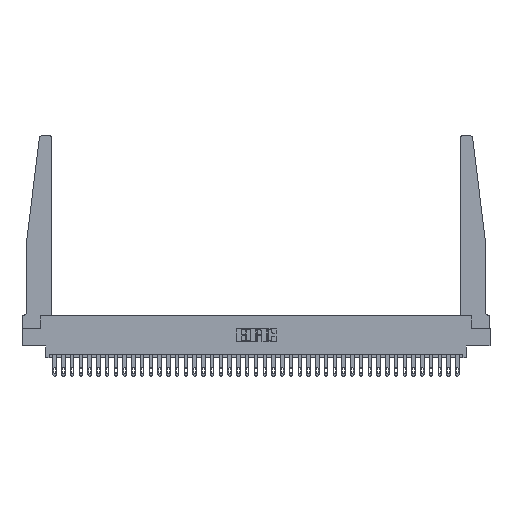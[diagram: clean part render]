
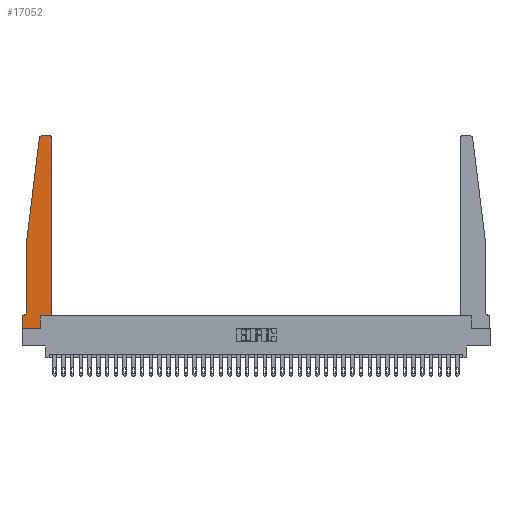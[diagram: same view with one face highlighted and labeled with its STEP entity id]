
A CAD part, top view. The second image highlights one B-rep face of the part: STEP entity #17052.
In plain terms, the highlighted planar face has unit normal (0, 0, 1).
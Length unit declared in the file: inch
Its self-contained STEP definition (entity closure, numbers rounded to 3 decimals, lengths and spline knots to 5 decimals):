
#277 = CARTESIAN_POINT ( 'NONE',  ( 0., 0.1875, 0.37 ) ) ;
#583 = CARTESIAN_POINT ( 'NONE',  ( 0., 0., 0.37 ) ) ;
#2379 = DIRECTION ( 'NONE',  ( 1., 0., 0. ) ) ;
#2888 = AXIS2_PLACEMENT_3D ( 'NONE', #5054, #20928, #2379 ) ;
#2895 = LINE ( 'NONE', #10766, #8839 ) ;
#2962 = EDGE_CURVE ( 'NONE', #16837, #6797, #2895, .T. ) ;
#3125 = VERTEX_POINT ( 'NONE', #22333 ) ;
#3218 = VERTEX_POINT ( 'NONE', #14650 ) ;
#3369 = DIRECTION ( 'NONE',  ( -1., 0., 0. ) ) ;
#3624 = EDGE_CURVE ( 'NONE', #3125, #34445, #22843, .T. ) ;
#4227 = LINE ( 'NONE', #7274, #10777 ) ;
#4383 = EDGE_CURVE ( 'NONE', #6797, #17259, #32723, .T. ) ;
#4899 = DIRECTION ( 'NONE',  ( 1., 0., 0. ) ) ;
#4927 = EDGE_CURVE ( 'NONE', #32567, #3218, #4227, .T. ) ;
#5054 = CARTESIAN_POINT ( 'NONE',  ( 0., 0.1875, 0.37 ) ) ;
#5168 = CARTESIAN_POINT ( 'NONE',  ( 0.015, 0.1875, 0.37 ) ) ;
#5901 = AXIS2_PLACEMENT_3D ( 'NONE', #31865, #12219, #31333 ) ;
#6479 = VECTOR ( 'NONE', #4899, 39.37008 ) ;
#6797 = VERTEX_POINT ( 'NONE', #9288 ) ;
#7006 = EDGE_CURVE ( 'NONE', #24190, #20669, #18581, .T. ) ;
#7035 = VECTOR ( 'NONE', #25612, 39.37008 ) ;
#7226 = CARTESIAN_POINT ( 'NONE',  ( 0.065, 1.25, 0.37 ) ) ;
#7274 = CARTESIAN_POINT ( 'NONE',  ( 0.25, 2.75, 0.37 ) ) ;
#7833 = ORIENTED_EDGE ( 'NONE', *, *, #18658, .T. ) ;
#8265 = AXIS2_PLACEMENT_3D ( 'NONE', #8854, #23119, #19753 ) ;
#8781 = EDGE_LOOP ( 'NONE', ( #22103, #17654, #23319, #31981, #24513, #7833, #25959, #12673, #13867, #21754, #24614, #31570 ) ) ;
#8839 = VECTOR ( 'NONE', #32549, 39.37008 ) ;
#8854 = CARTESIAN_POINT ( 'NONE',  ( 0.27653, 2.72, 0.37 ) ) ;
#9288 = CARTESIAN_POINT ( 'NONE',  ( 0.2605, 0., 0.37 ) ) ;
#10540 = CARTESIAN_POINT ( 'NONE',  ( 0.015, 0.2375, 0.37 ) ) ;
#10766 = CARTESIAN_POINT ( 'NONE',  ( 0., 0., 0.37 ) ) ;
#10777 = VECTOR ( 'NONE', #15133, 39.37008 ) ;
#12219 = DIRECTION ( 'NONE',  ( 0., 0., 1. ) ) ;
#12673 = ORIENTED_EDGE ( 'NONE', *, *, #2962, .T. ) ;
#12890 = EDGE_CURVE ( 'NONE', #15162, #16837, #29747, .T. ) ;
#13042 = CARTESIAN_POINT ( 'NONE',  ( 0.395, 2.75, 0.37 ) ) ;
#13258 = CARTESIAN_POINT ( 'NONE',  ( 0.2605, 0.18, 0.37 ) ) ;
#13793 = VECTOR ( 'NONE', #25829, 39.37008 ) ;
#13867 = ORIENTED_EDGE ( 'NONE', *, *, #4383, .T. ) ;
#14650 = CARTESIAN_POINT ( 'NONE',  ( 0.27653, 2.75, 0.37 ) ) ;
#14926 = CARTESIAN_POINT ( 'NONE',  ( 0.065, 1.25, 0.37 ) ) ;
#14945 = LINE ( 'NONE', #15122, #13793 ) ;
#15040 = VECTOR ( 'NONE', #29284, 39.37008 ) ;
#15122 = CARTESIAN_POINT ( 'NONE',  ( 0.065, 0.1875, 0.37 ) ) ;
#15133 = DIRECTION ( 'NONE',  ( -1., 0., 0. ) ) ;
#15162 = VERTEX_POINT ( 'NONE', #277 ) ;
#16837 = VERTEX_POINT ( 'NONE', #583 ) ;
#17052 = ADVANCED_FACE ( 'NONE', ( #29517 ), #20581, .T. ) ;
#17090 = VECTOR ( 'NONE', #24504, 39.37008 ) ;
#17259 = VERTEX_POINT ( 'NONE', #18975 ) ;
#17425 = LINE ( 'NONE', #14926, #28776 ) ;
#17654 = ORIENTED_EDGE ( 'NONE', *, *, #22647, .T. ) ;
#17788 = CARTESIAN_POINT ( 'NONE',  ( 0.24675, 2.72367, 0.37 ) ) ;
#18114 = LINE ( 'NONE', #7226, #7035 ) ;
#18581 = LINE ( 'NONE', #23205, #15040 ) ;
#18658 = EDGE_CURVE ( 'NONE', #34445, #15162, #14945, .T. ) ;
#18975 = CARTESIAN_POINT ( 'NONE',  ( 0.2605, 0.18, 0.37 ) ) ;
#19169 = EDGE_CURVE ( 'NONE', #17259, #24190, #32034, .T. ) ;
#19753 = DIRECTION ( 'NONE',  ( 1., 0., 0. ) ) ;
#19974 = DIRECTION ( 'NONE',  ( 0., 0., -1. ) ) ;
#20311 = EDGE_CURVE ( 'NONE', #34511, #3125, #18114, .T. ) ;
#20425 = EDGE_CURVE ( 'NONE', #20669, #32567, #25247, .T. ) ;
#20581 = PLANE ( 'NONE',  #2888 ) ;
#20669 = VERTEX_POINT ( 'NONE', #24692 ) ;
#20928 = DIRECTION ( 'NONE',  ( 0., 0., 1. ) ) ;
#21522 = CARTESIAN_POINT ( 'NONE',  ( 0., 0., 0.37 ) ) ;
#21666 = CARTESIAN_POINT ( 'NONE',  ( 0.425, 0.18, 0.37 ) ) ;
#21754 = ORIENTED_EDGE ( 'NONE', *, *, #19169, .T. ) ;
#22103 = ORIENTED_EDGE ( 'NONE', *, *, #4927, .T. ) ;
#22333 = CARTESIAN_POINT ( 'NONE',  ( 0.065, 0.2375, 0.37 ) ) ;
#22647 = EDGE_CURVE ( 'NONE', #3218, #26570, #23637, .T. ) ;
#22843 = CIRCLE ( 'NONE', #27419, 0.05 ) ;
#23119 = DIRECTION ( 'NONE',  ( 0., 0., 1. ) ) ;
#23205 = CARTESIAN_POINT ( 'NONE',  ( 0.425, 0.18, 0.37 ) ) ;
#23319 = ORIENTED_EDGE ( 'NONE', *, *, #24106, .T. ) ;
#23637 = CIRCLE ( 'NONE', #8265, 0.03 ) ;
#24106 = EDGE_CURVE ( 'NONE', #26570, #34511, #17425, .T. ) ;
#24190 = VERTEX_POINT ( 'NONE', #26863 ) ;
#24504 = DIRECTION ( 'NONE',  ( 0., 1., 0. ) ) ;
#24513 = ORIENTED_EDGE ( 'NONE', *, *, #3624, .T. ) ;
#24614 = ORIENTED_EDGE ( 'NONE', *, *, #7006, .T. ) ;
#24692 = CARTESIAN_POINT ( 'NONE',  ( 0.425, 2.72, 0.37 ) ) ;
#25247 = CIRCLE ( 'NONE', #5901, 0.03 ) ;
#25612 = DIRECTION ( 'NONE',  ( 0., -1., 0. ) ) ;
#25829 = DIRECTION ( 'NONE',  ( -1., 0., 0. ) ) ;
#25959 = ORIENTED_EDGE ( 'NONE', *, *, #12890, .T. ) ;
#26570 = VERTEX_POINT ( 'NONE', #17788 ) ;
#26863 = CARTESIAN_POINT ( 'NONE',  ( 0.425, 0.18, 0.37 ) ) ;
#27419 = AXIS2_PLACEMENT_3D ( 'NONE', #10540, #19974, #3369 ) ;
#28776 = VECTOR ( 'NONE', #30819, 39.37008 ) ;
#29284 = DIRECTION ( 'NONE',  ( 0., 1., 0. ) ) ;
#29517 = FACE_OUTER_BOUND ( 'NONE', #8781, .T. ) ;
#29747 = LINE ( 'NONE', #21522, #34107 ) ;
#30819 = DIRECTION ( 'NONE',  ( -0.122, -0.992, 0. ) ) ;
#31333 = DIRECTION ( 'NONE',  ( 1., 0., 0. ) ) ;
#31570 = ORIENTED_EDGE ( 'NONE', *, *, #20425, .T. ) ;
#31776 = CARTESIAN_POINT ( 'NONE',  ( 0.065, 1.25, 0.37 ) ) ;
#31865 = CARTESIAN_POINT ( 'NONE',  ( 0.395, 2.72, 0.37 ) ) ;
#31981 = ORIENTED_EDGE ( 'NONE', *, *, #20311, .T. ) ;
#32034 = LINE ( 'NONE', #21666, #6479 ) ;
#32069 = DIRECTION ( 'NONE',  ( 0., -1., 0. ) ) ;
#32549 = DIRECTION ( 'NONE',  ( 1., 0., 0. ) ) ;
#32567 = VERTEX_POINT ( 'NONE', #13042 ) ;
#32723 = LINE ( 'NONE', #13258, #17090 ) ;
#34107 = VECTOR ( 'NONE', #32069, 39.37008 ) ;
#34445 = VERTEX_POINT ( 'NONE', #5168 ) ;
#34511 = VERTEX_POINT ( 'NONE', #31776 ) ;
